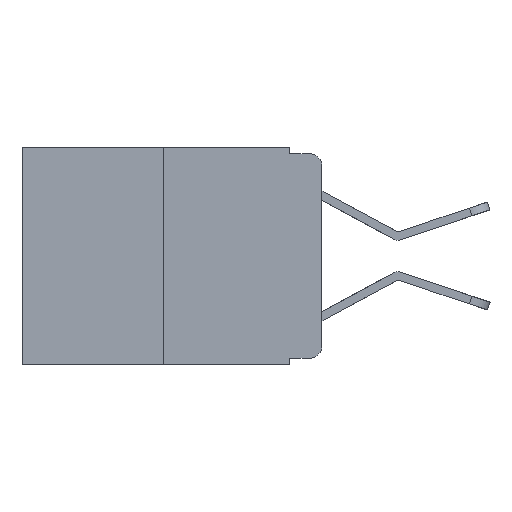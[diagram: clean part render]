
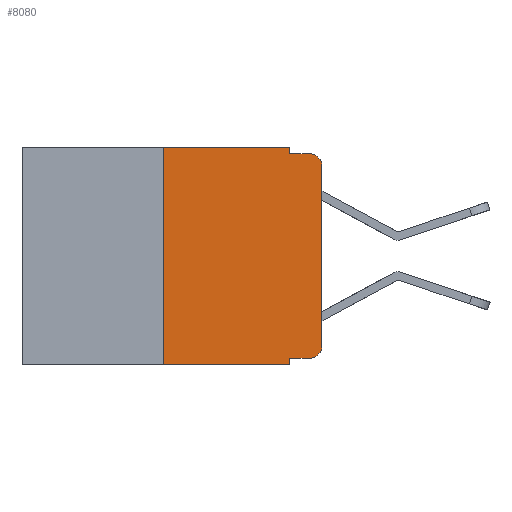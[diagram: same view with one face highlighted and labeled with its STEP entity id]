
A CAD part, left-side view. The second image highlights one B-rep face of the part: STEP entity #8080.
In plain terms, the highlighted planar face has unit normal (-1, 0, 0).
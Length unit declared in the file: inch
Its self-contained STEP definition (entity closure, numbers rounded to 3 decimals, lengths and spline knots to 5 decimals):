
#129 = EDGE_CURVE ( 'NONE', #9182, #3741, #15214, .T. ) ;
#338 = ORIENTED_EDGE ( 'NONE', *, *, #15838, .F. ) ;
#822 = EDGE_CURVE ( 'NONE', #10182, #16252, #7154, .T. ) ;
#849 = EDGE_CURVE ( 'NONE', #7442, #12387, #6265, .T. ) ;
#1404 = CARTESIAN_POINT ( 'NONE',  ( 0., 0.25, 0. ) ) ;
#1463 = EDGE_CURVE ( 'NONE', #16961, #12387, #3026, .T. ) ;
#1548 = VECTOR ( 'NONE', #2826, 39.37008 ) ;
#1619 = EDGE_CURVE ( 'NONE', #16252, #7442, #17384, .T. ) ;
#1841 = CARTESIAN_POINT ( 'NONE',  ( 0., 0.051, -0.343 ) ) ;
#1905 = CARTESIAN_POINT ( 'NONE',  ( 0., 0.051, -0.01 ) ) ;
#2341 = DIRECTION ( 'NONE',  ( 0., 0., 1. ) ) ;
#2359 = ORIENTED_EDGE ( 'NONE', *, *, #1463, .F. ) ;
#2770 = EDGE_CURVE ( 'NONE', #9182, #15391, #3029, .T. ) ;
#2826 = DIRECTION ( 'NONE',  ( 0., -1., 0. ) ) ;
#2994 = ORIENTED_EDGE ( 'NONE', *, *, #129, .F. ) ;
#3026 = LINE ( 'NONE', #9801, #8344 ) ;
#3029 = LINE ( 'NONE', #3208, #15617 ) ;
#3208 = CARTESIAN_POINT ( 'NONE',  ( 0., 0.473, -0.343 ) ) ;
#3318 = VECTOR ( 'NONE', #5993, 39.37008 ) ;
#3741 = VERTEX_POINT ( 'NONE', #5715 ) ;
#4012 = CARTESIAN_POINT ( 'NONE',  ( 0., 0.051, -0.333 ) ) ;
#4406 = DIRECTION ( 'NONE',  ( 0., -1., 0. ) ) ;
#5250 = CARTESIAN_POINT ( 'NONE',  ( 0., 0.02, -0.313 ) ) ;
#5385 = CARTESIAN_POINT ( 'NONE',  ( 0., 0.473, 0. ) ) ;
#5410 = AXIS2_PLACEMENT_3D ( 'NONE', #10795, #16246, #6702 ) ;
#5715 = CARTESIAN_POINT ( 'NONE',  ( 0., 0.25, 0. ) ) ;
#5993 = DIRECTION ( 'NONE',  ( 0., -1., 0. ) ) ;
#6016 = CARTESIAN_POINT ( 'NONE',  ( 0., 0., -0.03 ) ) ;
#6161 = CARTESIAN_POINT ( 'NONE',  ( 0., 0., -0.313 ) ) ;
#6181 = CARTESIAN_POINT ( 'NONE',  ( 0., 0.051, 0. ) ) ;
#6237 = CARTESIAN_POINT ( 'NONE',  ( 0., 0.051, -0.333 ) ) ;
#6265 = CIRCLE ( 'NONE', #5410, 0.02 ) ;
#6464 = ORIENTED_EDGE ( 'NONE', *, *, #1619, .T. ) ;
#6702 = DIRECTION ( 'NONE',  ( 0., 0., -1. ) ) ;
#6901 = CARTESIAN_POINT ( 'NONE',  ( 0., 0.02, -0.333 ) ) ;
#7125 = EDGE_CURVE ( 'NONE', #3741, #12101, #15363, .T. ) ;
#7154 = CIRCLE ( 'NONE', #15553, 0.02 ) ;
#7222 = CARTESIAN_POINT ( 'NONE',  ( 0., 0.02, -0.01 ) ) ;
#7229 = DIRECTION ( 'NONE',  ( 0., 0., 1. ) ) ;
#7442 = VERTEX_POINT ( 'NONE', #6016 ) ;
#7478 = EDGE_LOOP ( 'NONE', ( #6464, #13364, #2359, #16004, #8704, #2994, #15266, #338, #13680, #17858 ) ) ;
#8080 = ADVANCED_FACE ( 'NONE', ( #15481 ), #9548, .F. ) ;
#8344 = VECTOR ( 'NONE', #13879, 39.37008 ) ;
#8441 = LINE ( 'NONE', #12786, #13265 ) ;
#8609 = VECTOR ( 'NONE', #17380, 39.37008 ) ;
#8704 = ORIENTED_EDGE ( 'NONE', *, *, #7125, .F. ) ;
#9053 = CARTESIAN_POINT ( 'NONE',  ( 0., 0.051, 0. ) ) ;
#9182 = VERTEX_POINT ( 'NONE', #9528 ) ;
#9528 = CARTESIAN_POINT ( 'NONE',  ( 0., 0.25, -0.343 ) ) ;
#9548 = PLANE ( 'NONE',  #17839 ) ;
#9801 = CARTESIAN_POINT ( 'NONE',  ( 0., 0.051, -0.01 ) ) ;
#9960 = DIRECTION ( 'NONE',  ( 1., 0., 0. ) ) ;
#10182 = VERTEX_POINT ( 'NONE', #6901 ) ;
#10795 = CARTESIAN_POINT ( 'NONE',  ( 0., 0.02, -0.03 ) ) ;
#11737 = VERTEX_POINT ( 'NONE', #6237 ) ;
#12101 = VERTEX_POINT ( 'NONE', #9053 ) ;
#12387 = VERTEX_POINT ( 'NONE', #7222 ) ;
#12462 = DIRECTION ( 'NONE',  ( -1., 0., 0. ) ) ;
#12786 = CARTESIAN_POINT ( 'NONE',  ( 0., 0.051, 0. ) ) ;
#13265 = VECTOR ( 'NONE', #15661, 39.37008 ) ;
#13364 = ORIENTED_EDGE ( 'NONE', *, *, #849, .T. ) ;
#13680 = ORIENTED_EDGE ( 'NONE', *, *, #14420, .T. ) ;
#13879 = DIRECTION ( 'NONE',  ( 0., -1., 0. ) ) ;
#14286 = LINE ( 'NONE', #6181, #8609 ) ;
#14420 = EDGE_CURVE ( 'NONE', #11737, #10182, #15704, .T. ) ;
#14807 = CARTESIAN_POINT ( 'NONE',  ( 0., 0., 0. ) ) ;
#15069 = CARTESIAN_POINT ( 'NONE',  ( 0., 0.473, 0. ) ) ;
#15153 = DIRECTION ( 'NONE',  ( 0., 0., -1. ) ) ;
#15214 = LINE ( 'NONE', #1404, #16086 ) ;
#15266 = ORIENTED_EDGE ( 'NONE', *, *, #2770, .T. ) ;
#15363 = LINE ( 'NONE', #5385, #1548 ) ;
#15391 = VERTEX_POINT ( 'NONE', #1841 ) ;
#15481 = FACE_OUTER_BOUND ( 'NONE', #7478, .T. ) ;
#15553 = AXIS2_PLACEMENT_3D ( 'NONE', #5250, #12462, #17714 ) ;
#15617 = VECTOR ( 'NONE', #4406, 39.37008 ) ;
#15661 = DIRECTION ( 'NONE',  ( 0., 0., -1. ) ) ;
#15704 = LINE ( 'NONE', #4012, #3318 ) ;
#15838 = EDGE_CURVE ( 'NONE', #11737, #15391, #14286, .T. ) ;
#16004 = ORIENTED_EDGE ( 'NONE', *, *, #16610, .F. ) ;
#16086 = VECTOR ( 'NONE', #7229, 39.37008 ) ;
#16154 = VECTOR ( 'NONE', #2341, 39.37008 ) ;
#16246 = DIRECTION ( 'NONE',  ( -1., 0., 0. ) ) ;
#16252 = VERTEX_POINT ( 'NONE', #6161 ) ;
#16610 = EDGE_CURVE ( 'NONE', #12101, #16961, #8441, .T. ) ;
#16961 = VERTEX_POINT ( 'NONE', #1905 ) ;
#17380 = DIRECTION ( 'NONE',  ( 0., 0., -1. ) ) ;
#17384 = LINE ( 'NONE', #14807, #16154 ) ;
#17714 = DIRECTION ( 'NONE',  ( 0., 0., -1. ) ) ;
#17839 = AXIS2_PLACEMENT_3D ( 'NONE', #15069, #9960, #15153 ) ;
#17858 = ORIENTED_EDGE ( 'NONE', *, *, #822, .T. ) ;
